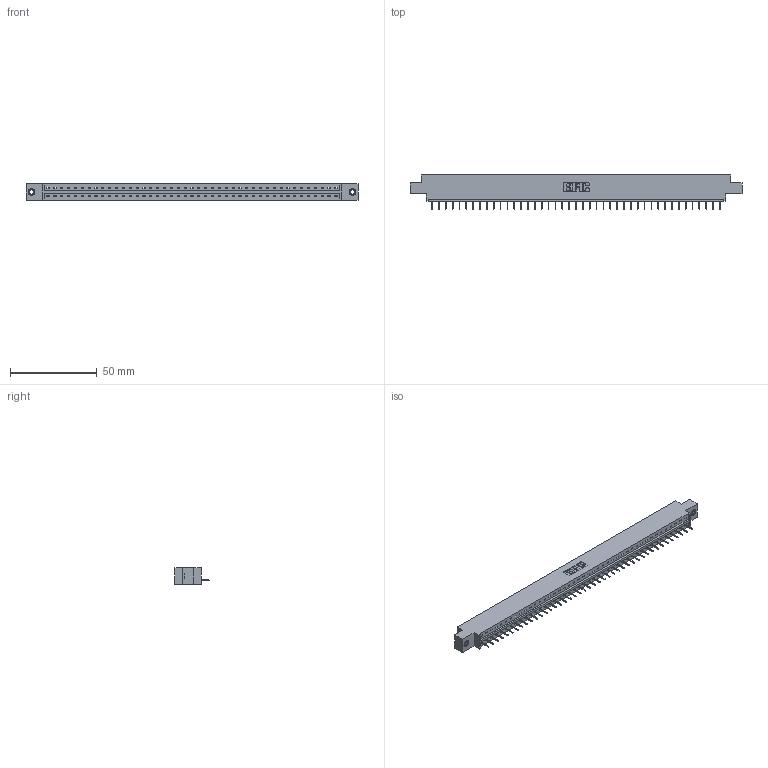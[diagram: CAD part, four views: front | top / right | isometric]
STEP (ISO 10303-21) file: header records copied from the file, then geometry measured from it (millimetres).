
FILE_DESCRIPTION (( 'STEP AP203' ), '1' );
FILE_NAME ('833-043-524-607.STEP', '2020-06-03T23:42:47', ( '' ), ( '' ), 'SwSTEP 2.0', 'SolidWorks 2020', '' );
FILE_SCHEMA (( 'CONFIG_CONTROL_DESIGN' ));
Length unit declared in the file: inch
Products named in the file (4): 833 Part_Offset - .156 Dia - TI; 833-043-524-607; 345-292-001_345-293-124; 345-250-001_345-250-005-103
Assembly tree (46 placements, depth 2):
  833-043-524-607
    833 Part_Offset - .156 Dia - TI
    345-292-001_345-293-124  x43
    345-250-001_345-250-005-103  x2
Bounding box: 191.92 x 19.69 x 9.4 mm (x, y, z)
Volume: 18910.2 mm3; surface area: 20118.9 mm2
Topology: 46 solids, 46 shells, 2844 faces, 8199 edges, 5286 vertices
Faces by surface type: plane 2170, cylinder 658, cone 12, torus 4
Entity records: 27550 total; most frequent: CARTESIAN_POINT 4734, ORIENTED_EDGE 4706, DIRECTION 4025, EDGE_CURVE 2353, VECTOR 2209, LINE 2209, VERTEX_POINT 1560, AXIS2_PLACEMENT_3D 908
